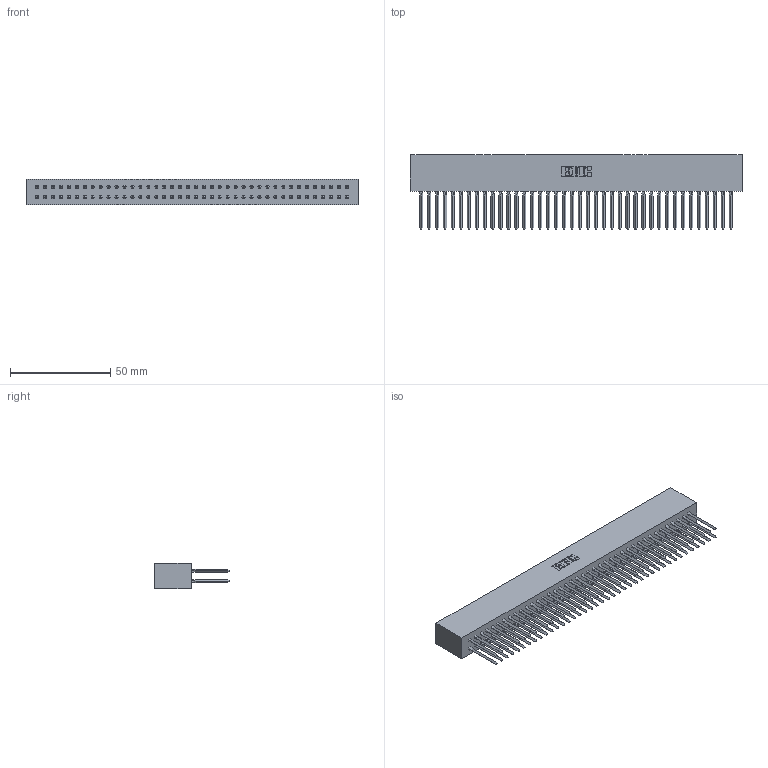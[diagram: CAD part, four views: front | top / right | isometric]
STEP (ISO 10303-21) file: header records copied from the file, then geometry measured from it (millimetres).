
FILE_DESCRIPTION (( 'STEP AP203' ), '1' );
FILE_NAME ('317-080-542-801.STEP', '2020-02-28T09:12:56', ( '' ), ( '' ), 'SwSTEP 2.0', 'SolidWorks 2016', '' );
FILE_SCHEMA (( 'CONFIG_CONTROL_DESIGN' ));
Length unit declared in the file: inch
Products named in the file (3): 317-080-542-801; 317-290-003_542; 317 Part_Lugless
Assembly tree (81 placements, depth 2):
  317-080-542-801
    317 Part_Lugless
    317-290-003_542  x80
Bounding box: 165.71 x 37.34 x 12.7 mm (x, y, z)
Volume: 28801.5 mm3; surface area: 40163.6 mm2
Topology: 81 solids, 81 shells, 4650 faces, 13039 edges, 8318 vertices
Faces by surface type: plane 3730, cylinder 600, bspline 320
Entity records: 56707 total; most frequent: CARTESIAN_POINT 10141, ORIENTED_EDGE 9804, DIRECTION 8242, EDGE_CURVE 4902, LINE 4740, VECTOR 4740, VERTEX_POINT 3262, AXIS2_PLACEMENT_3D 1751
